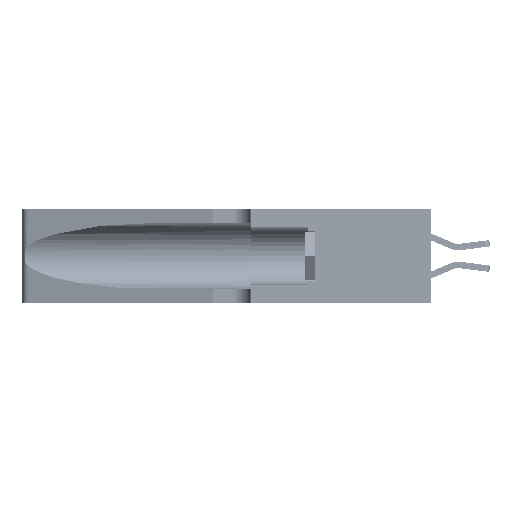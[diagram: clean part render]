
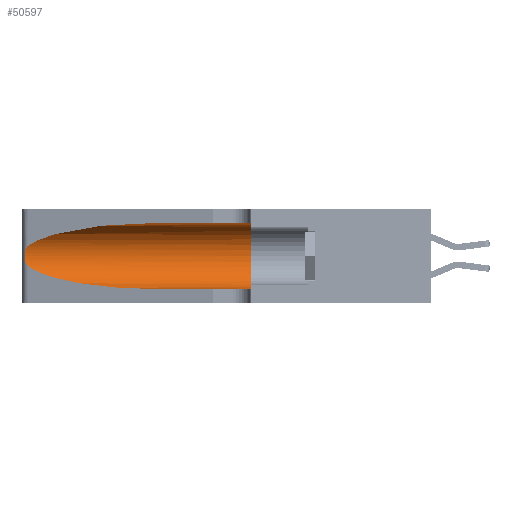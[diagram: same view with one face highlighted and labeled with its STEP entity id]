
A CAD part, left-side view. The second image highlights one B-rep face of the part: STEP entity #50597.
In plain terms, the highlighted cylindrical face has radius 3.308 mm (diameter 6.617 mm), a partial arc.
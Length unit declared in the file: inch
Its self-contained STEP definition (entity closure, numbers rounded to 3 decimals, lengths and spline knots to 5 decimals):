
#3310 = CARTESIAN_POINT ( 'NONE',  ( 0.26075, 1.23896, 0.19203 ) ) ;
#3713 = LINE ( 'NONE', #25946, #13649 ) ;
#4062 = ORIENTED_EDGE ( 'NONE', *, *, #31260, .T. ) ;
#4248 = VERTEX_POINT ( 'NONE', #53185 ) ;
#4288 =( BOUNDED_CURVE ( )  B_SPLINE_CURVE ( 3, ( #7376, #32391, #52878, #36521 ),
 .UNSPECIFIED., .F., .T. ) 
 B_SPLINE_CURVE_WITH_KNOTS ( ( 4, 4 ),
 ( 1.5708, 2.84003 ),
 .UNSPECIFIED. ) 
 CURVE ( )  GEOMETRIC_REPRESENTATION_ITEM ( )  RATIONAL_B_SPLINE_CURVE ( ( 1., 0.87, 0.87, 1. ) ) 
 REPRESENTATION_ITEM ( '' )  );
#4408 = CARTESIAN_POINT ( 'NONE',  ( 0.1305, 0.72297, 0.31525 ) ) ;
#5045 = DIRECTION ( 'NONE',  ( 0., -1., 0. ) ) ;
#6604 = EDGE_LOOP ( 'NONE', ( #26714, #45613, #4062, #6885, #12703, #27662 ) ) ;
#6885 = ORIENTED_EDGE ( 'NONE', *, *, #38837, .T. ) ;
#7376 = CARTESIAN_POINT ( 'NONE',  ( 0.1305, 0.72297, 0.31525 ) ) ;
#7554 = CARTESIAN_POINT ( 'NONE',  ( 0.26017, 1.23833, 0.17102 ) ) ;
#8823 = CARTESIAN_POINT ( 'NONE',  ( 0.1305, 0.72297, 0.05475 ) ) ;
#9591 = VERTEX_POINT ( 'NONE', #38147 ) ;
#10328 = AXIS2_PLACEMENT_3D ( 'NONE', #45427, #20672, #49575 ) ;
#10677 = VERTEX_POINT ( 'NONE', #33034 ) ;
#11633 = VERTEX_POINT ( 'NONE', #26089 ) ;
#11643 = CARTESIAN_POINT ( 'NONE',  ( 0.25487, 1.22718, 0.22369 ) ) ;
#11811 = CARTESIAN_POINT ( 'NONE',  ( 0.25789, 1.23486, 0.15765 ) ) ;
#12340 = FACE_OUTER_BOUND ( 'NONE', #6604, .T. ) ;
#12435 = EDGE_CURVE ( 'NONE', #10677, #9591, #25291, .T. ) ;
#12703 = ORIENTED_EDGE ( 'NONE', *, *, #12435, .F. ) ;
#12918 = VECTOR ( 'NONE', #27252, 39.37008 ) ;
#13620 = AXIS2_PLACEMENT_3D ( 'NONE', #46900, #38615, #13816 ) ;
#13649 = VECTOR ( 'NONE', #5045, 39.37008 ) ;
#13816 = DIRECTION ( 'NONE',  ( 0., 0., -1. ) ) ;
#16060 = CARTESIAN_POINT ( 'NONE',  ( 0.25555, 1.22993, 0.14849 ) ) ;
#18381 = EDGE_CURVE ( 'NONE', #27968, #35887, #4288, .T. ) ;
#20672 = DIRECTION ( 'NONE',  ( 0., 1., 0. ) ) ;
#23053 = CARTESIAN_POINT ( 'NONE',  ( 0.1305, 1.61858, 0.05475 ) ) ;
#24234 = CARTESIAN_POINT ( 'NONE',  ( 0.25787, 1.23484, 0.2124 ) ) ;
#25291 = CIRCLE ( 'NONE', #10328, 0.13025 ) ;
#25493 = CARTESIAN_POINT ( 'NONE',  ( 0.25487, 1.22718, 0.14631 ) ) ;
#25946 = CARTESIAN_POINT ( 'NONE',  ( 0.1305, 1.61858, 0.31525 ) ) ;
#26089 = CARTESIAN_POINT ( 'NONE',  ( 0.25487, 1.22718, 0.14631 ) ) ;
#26714 = ORIENTED_EDGE ( 'NONE', *, *, #18381, .T. ) ;
#27252 = DIRECTION ( 'NONE',  ( 0., -1., 0. ) ) ;
#27662 = ORIENTED_EDGE ( 'NONE', *, *, #29279, .F. ) ;
#27968 = VERTEX_POINT ( 'NONE', #4408 ) ;
#28414 = CARTESIAN_POINT ( 'NONE',  ( 0.26018, 1.23835, 0.19895 ) ) ;
#29279 = EDGE_CURVE ( 'NONE', #27968, #10677, #3713, .T. ) ;
#31260 = EDGE_CURVE ( 'NONE', #11633, #4248, #44624, .T. ) ;
#32387 = CARTESIAN_POINT ( 'NONE',  ( 0.25555, 1.22994, 0.2215 ) ) ;
#32391 = CARTESIAN_POINT ( 'NONE',  ( 0.18966, 0.96281, 0.31525 ) ) ;
#32561 = CARTESIAN_POINT ( 'NONE',  ( 0.26075, 1.23896, 0.178 ) ) ;
#33034 = CARTESIAN_POINT ( 'NONE',  ( 0.1305, 0.35, 0.31525 ) ) ;
#33164 = CYLINDRICAL_SURFACE ( 'NONE', #13620, 0.13025 ) ;
#33809 = CARTESIAN_POINT ( 'NONE',  ( 0.18966, 0.96281, 0.05475 ) ) ;
#35612 = B_SPLINE_CURVE_WITH_KNOTS ( 'NONE', 3,
 ( #11643, #32387, #48923, #24234, #53050, #28414, #3310, #32561, #7554, #36692, #11811, #40834, #16060, #44955 ),
 .UNSPECIFIED., .F., .F.,
 ( 4, 2, 2, 2, 2, 2, 4 ),
 ( 0., 0.00027, 0.00053, 0.00107, 0.0016, 0.00187, 0.00214 ),
 .UNSPECIFIED. ) ;
#35887 = VERTEX_POINT ( 'NONE', #48274 ) ;
#36521 = CARTESIAN_POINT ( 'NONE',  ( 0.25487, 1.22718, 0.22369 ) ) ;
#36692 = CARTESIAN_POINT ( 'NONE',  ( 0.25856, 1.23593, 0.16098 ) ) ;
#38147 = CARTESIAN_POINT ( 'NONE',  ( 0.1305, 0.35, 0.05475 ) ) ;
#38615 = DIRECTION ( 'NONE',  ( 0., -1., 0. ) ) ;
#38837 = EDGE_CURVE ( 'NONE', #4248, #9591, #45950, .T. ) ;
#40834 = CARTESIAN_POINT ( 'NONE',  ( 0.25639, 1.23186, 0.15144 ) ) ;
#42855 = EDGE_CURVE ( 'NONE', #35887, #11633, #35612, .T. ) ;
#44624 =( BOUNDED_CURVE ( )  B_SPLINE_CURVE ( 3, ( #25493, #46036, #33809, #8823 ),
 .UNSPECIFIED., .F., .T. ) 
 B_SPLINE_CURVE_WITH_KNOTS ( ( 4, 4 ),
 ( 3.44316, 4.71239 ),
 .UNSPECIFIED. ) 
 CURVE ( )  GEOMETRIC_REPRESENTATION_ITEM ( )  RATIONAL_B_SPLINE_CURVE ( ( 1., 0.87, 0.87, 1. ) ) 
 REPRESENTATION_ITEM ( '' )  );
#44955 = CARTESIAN_POINT ( 'NONE',  ( 0.25487, 1.22718, 0.14631 ) ) ;
#45427 = CARTESIAN_POINT ( 'NONE',  ( 0.1305, 0.35, 0.185 ) ) ;
#45613 = ORIENTED_EDGE ( 'NONE', *, *, #42855, .T. ) ;
#45950 = LINE ( 'NONE', #23053, #12918 ) ;
#46036 = CARTESIAN_POINT ( 'NONE',  ( 0.2373, 1.15595, 0.08982 ) ) ;
#46900 = CARTESIAN_POINT ( 'NONE',  ( 0.1305, 1.61858, 0.185 ) ) ;
#48274 = CARTESIAN_POINT ( 'NONE',  ( 0.25487, 1.22718, 0.22369 ) ) ;
#48923 = CARTESIAN_POINT ( 'NONE',  ( 0.25639, 1.23184, 0.21858 ) ) ;
#49575 = DIRECTION ( 'NONE',  ( 0., 0., 1. ) ) ;
#50597 = ADVANCED_FACE ( 'NONE', ( #12340 ), #33164, .F. ) ;
#52878 = CARTESIAN_POINT ( 'NONE',  ( 0.2373, 1.15595, 0.28018 ) ) ;
#53050 = CARTESIAN_POINT ( 'NONE',  ( 0.25854, 1.2359, 0.20912 ) ) ;
#53185 = CARTESIAN_POINT ( 'NONE',  ( 0.1305, 0.72297, 0.05475 ) ) ;
